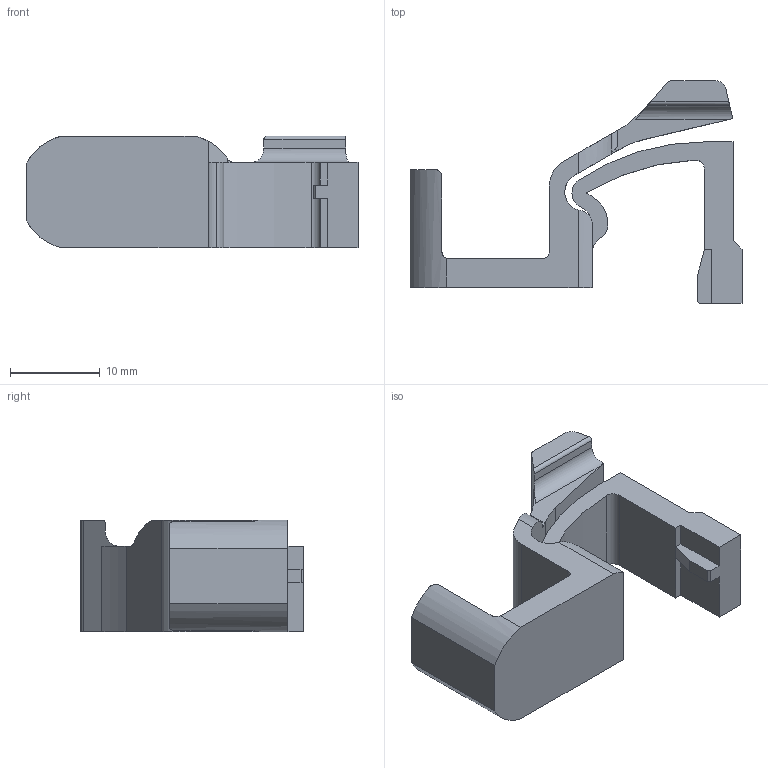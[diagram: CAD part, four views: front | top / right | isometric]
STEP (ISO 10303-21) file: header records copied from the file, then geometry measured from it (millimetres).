
FILE_DESCRIPTION(/* description */ (''),/* implementation_level */ '2;1');
FILE_NAME(/* name */ 'ChoosyBoogle v3 3.stp',/* time_stamp */ '2022-11-09T21:44:44-05:00',/* author */ ('Author'),/* organization */ (''),/* preprocessor_version */ 'ST-DEVELOPER v18.1',/* originating_system */ 'Autodesk Inventor 2022',/* authorisation */ '');
FILE_SCHEMA (('AUTOMOTIVE_DESIGN { 1 0 10303 214 3 1 1 }'));
Length unit declared in the file: metre
Products named in the file (1): ChoosyBoogle v3
Bounding box: 36.92 x 24.74 x 12.45 mm (x, y, z)
Volume: 3226.1 mm3; surface area: 2832.1 mm2
Topology: 1 solids, 1 shells, 63 faces, 180 edges, 120 vertices
Faces by surface type: plane 34, cylinder 29
Entity records: 2170 total; most frequent: CARTESIAN_POINT 421, ORIENTED_EDGE 360, DIRECTION 355, EDGE_CURVE 180, LINE 119, VECTOR 119, VERTEX_POINT 119, AXIS2_PLACEMENT_3D 118
